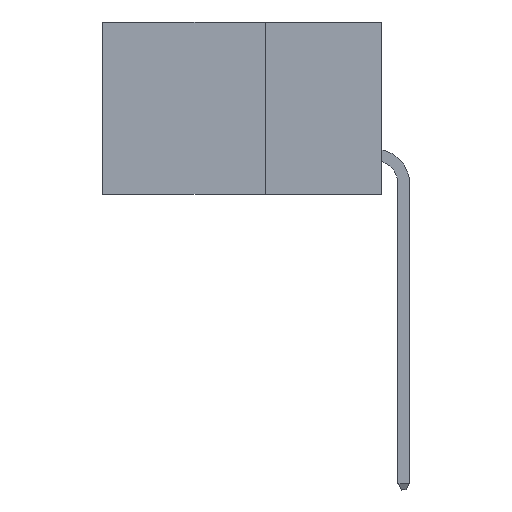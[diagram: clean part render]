
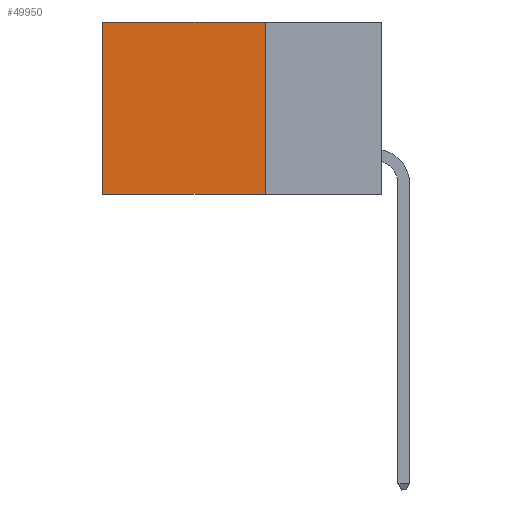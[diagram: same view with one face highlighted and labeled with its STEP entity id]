
A CAD part, left-side view. The second image highlights one B-rep face of the part: STEP entity #49950.
In plain terms, the highlighted planar face has unit normal (-1, 0, 0).
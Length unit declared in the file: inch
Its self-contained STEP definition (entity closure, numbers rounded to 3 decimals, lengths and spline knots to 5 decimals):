
#640 = VERTEX_POINT ( 'NONE', #25473 ) ;
#1662 = FACE_OUTER_BOUND ( 'NONE', #11844, .T. ) ;
#2741 = VERTEX_POINT ( 'NONE', #14352 ) ;
#3364 = DIRECTION ( 'NONE',  ( 0., 1., 0. ) ) ;
#7269 = LINE ( 'NONE', #23637, #40806 ) ;
#8837 = DIRECTION ( 'NONE',  ( 0., 0., -1. ) ) ;
#9548 = EDGE_CURVE ( 'NONE', #640, #12205, #26683, .T. ) ;
#11711 = VECTOR ( 'NONE', #39401, 39.37008 ) ;
#11844 = EDGE_LOOP ( 'NONE', ( #39703, #31459, #16098, #23861 ) ) ;
#12205 = VERTEX_POINT ( 'NONE', #34938 ) ;
#13474 = CARTESIAN_POINT ( 'NONE',  ( 0.2875, 0.6, 0. ) ) ;
#14352 = CARTESIAN_POINT ( 'NONE',  ( 0.2875, 0.6, -0.37 ) ) ;
#15714 = DIRECTION ( 'NONE',  ( 0., 1., 0. ) ) ;
#15837 = PLANE ( 'NONE',  #46748 ) ;
#16098 = ORIENTED_EDGE ( 'NONE', *, *, #9548, .F. ) ;
#18465 = CARTESIAN_POINT ( 'NONE',  ( 0.2875, 0.25, 0. ) ) ;
#23637 = CARTESIAN_POINT ( 'NONE',  ( 0.2875, 0.25, -0.37 ) ) ;
#23773 = LINE ( 'NONE', #43743, #11711 ) ;
#23861 = ORIENTED_EDGE ( 'NONE', *, *, #32572, .T. ) ;
#25473 = CARTESIAN_POINT ( 'NONE',  ( 0.2875, 0.25, 0. ) ) ;
#25559 = EDGE_CURVE ( 'NONE', #46642, #2741, #23773, .T. ) ;
#26683 = LINE ( 'NONE', #41560, #42489 ) ;
#31459 = ORIENTED_EDGE ( 'NONE', *, *, #33968, .F. ) ;
#32137 = CARTESIAN_POINT ( 'NONE',  ( 0.2875, 0.25, 0. ) ) ;
#32572 = EDGE_CURVE ( 'NONE', #640, #46642, #45623, .T. ) ;
#33968 = EDGE_CURVE ( 'NONE', #12205, #2741, #7269, .T. ) ;
#34938 = CARTESIAN_POINT ( 'NONE',  ( 0.2875, 0.25, -0.37 ) ) ;
#39401 = DIRECTION ( 'NONE',  ( 0., 0., -1. ) ) ;
#39703 = ORIENTED_EDGE ( 'NONE', *, *, #25559, .T. ) ;
#40806 = VECTOR ( 'NONE', #15714, 39.37008 ) ;
#40846 = DIRECTION ( 'NONE',  ( 1., 0., 0. ) ) ;
#41560 = CARTESIAN_POINT ( 'NONE',  ( 0.2875, 0.25, 0. ) ) ;
#42321 = DIRECTION ( 'NONE',  ( 0., 0., -1. ) ) ;
#42489 = VECTOR ( 'NONE', #42321, 39.37008 ) ;
#43743 = CARTESIAN_POINT ( 'NONE',  ( 0.2875, 0.6, 0. ) ) ;
#45623 = LINE ( 'NONE', #18465, #46491 ) ;
#46491 = VECTOR ( 'NONE', #3364, 39.37008 ) ;
#46642 = VERTEX_POINT ( 'NONE', #13474 ) ;
#46748 = AXIS2_PLACEMENT_3D ( 'NONE', #32137, #40846, #8837 ) ;
#49950 = ADVANCED_FACE ( 'NONE', ( #1662 ), #15837, .F. ) ;
